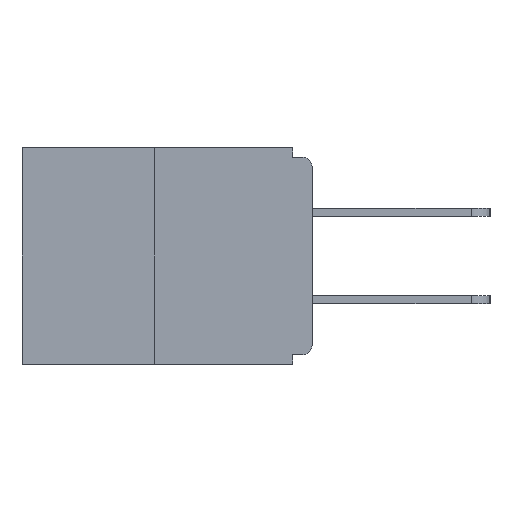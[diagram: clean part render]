
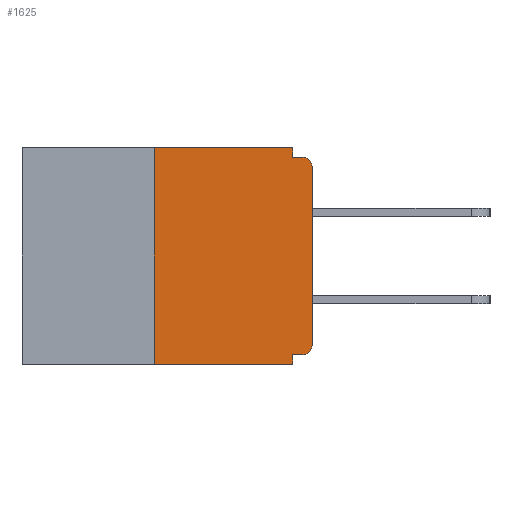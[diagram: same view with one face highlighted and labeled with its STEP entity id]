
A CAD part, left-side view. The second image highlights one B-rep face of the part: STEP entity #1625.
In plain terms, the highlighted planar face has unit normal (-1, 0, 0).
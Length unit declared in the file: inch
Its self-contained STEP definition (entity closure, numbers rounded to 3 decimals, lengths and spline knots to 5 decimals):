
#5 = AXIS2_PLACEMENT_3D ( 'NONE', #1478, #8790, #7945 ) ;
#164 = VECTOR ( 'NONE', #8709, 39.37008 ) ;
#297 = LINE ( 'NONE', #11560, #9770 ) ;
#330 = CARTESIAN_POINT ( 'NONE',  ( 0., 0.25, -0.343 ) ) ;
#506 = VECTOR ( 'NONE', #2333, 39.37008 ) ;
#747 = VERTEX_POINT ( 'NONE', #11713 ) ;
#1061 = CARTESIAN_POINT ( 'NONE',  ( 0., 0.031, 0. ) ) ;
#1192 = CARTESIAN_POINT ( 'NONE',  ( 0., 0.015, -0.313 ) ) ;
#1351 = DIRECTION ( 'NONE',  ( 0., 0., 1. ) ) ;
#1478 = CARTESIAN_POINT ( 'NONE',  ( 0., 0.46, 0. ) ) ;
#1625 = ADVANCED_FACE ( 'NONE', ( #10551 ), #2191, .F. ) ;
#1635 = EDGE_CURVE ( 'NONE', #10508, #9556, #4396, .T. ) ;
#1732 = EDGE_CURVE ( 'NONE', #10364, #5796, #297, .T. ) ;
#1770 = EDGE_CURVE ( 'NONE', #5796, #747, #4181, .T. ) ;
#2173 = CARTESIAN_POINT ( 'NONE',  ( 0., 0., -0.328 ) ) ;
#2191 = PLANE ( 'NONE',  #5 ) ;
#2203 = DIRECTION ( 'NONE',  ( -1., 0., 0. ) ) ;
#2333 = DIRECTION ( 'NONE',  ( 0., -1., 0. ) ) ;
#2385 = CIRCLE ( 'NONE', #3737, 0.015 ) ;
#2574 = LINE ( 'NONE', #2173, #9597 ) ;
#2577 = CARTESIAN_POINT ( 'NONE',  ( 0., 0., -0.015 ) ) ;
#2754 = VECTOR ( 'NONE', #9348, 39.37008 ) ;
#3323 = VERTEX_POINT ( 'NONE', #9105 ) ;
#3351 = EDGE_CURVE ( 'NONE', #7795, #10508, #2574, .T. ) ;
#3388 = CARTESIAN_POINT ( 'NONE',  ( 0., 0.46, -0.343 ) ) ;
#3415 = CARTESIAN_POINT ( 'NONE',  ( 0., 0.031, -0.343 ) ) ;
#3664 = ORIENTED_EDGE ( 'NONE', *, *, #5483, .T. ) ;
#3737 = AXIS2_PLACEMENT_3D ( 'NONE', #10527, #2203, #10576 ) ;
#3806 = VECTOR ( 'NONE', #10780, 39.37008 ) ;
#3870 = EDGE_CURVE ( 'NONE', #7795, #3323, #8283, .T. ) ;
#4018 = VECTOR ( 'NONE', #10853, 39.37008 ) ;
#4101 = CARTESIAN_POINT ( 'NONE',  ( 0., 0.031, -0.343 ) ) ;
#4181 = LINE ( 'NONE', #2577, #4018 ) ;
#4396 = LINE ( 'NONE', #4101, #164 ) ;
#4628 = ORIENTED_EDGE ( 'NONE', *, *, #3870, .T. ) ;
#4729 = DIRECTION ( 'NONE',  ( 0., 0., -1. ) ) ;
#5066 = CARTESIAN_POINT ( 'NONE',  ( 0., 0.25, 0. ) ) ;
#5091 = CARTESIAN_POINT ( 'NONE',  ( 0., 0.46, 0. ) ) ;
#5300 = EDGE_LOOP ( 'NONE', ( #7437, #8618, #5725, #10339, #7276, #4628, #11857, #3664, #6921, #9392 ) ) ;
#5483 = EDGE_CURVE ( 'NONE', #10702, #747, #2385, .T. ) ;
#5725 = ORIENTED_EDGE ( 'NONE', *, *, #8957, .T. ) ;
#5796 = VERTEX_POINT ( 'NONE', #8775 ) ;
#6315 = LINE ( 'NONE', #7747, #6838 ) ;
#6353 = EDGE_CURVE ( 'NONE', #9298, #10775, #6315, .T. ) ;
#6661 = CARTESIAN_POINT ( 'NONE',  ( 0., 0., -0.03 ) ) ;
#6838 = VECTOR ( 'NONE', #1351, 39.37008 ) ;
#6921 = ORIENTED_EDGE ( 'NONE', *, *, #1770, .F. ) ;
#7130 = CARTESIAN_POINT ( 'NONE',  ( 0., 0.015, -0.328 ) ) ;
#7276 = ORIENTED_EDGE ( 'NONE', *, *, #3351, .F. ) ;
#7437 = ORIENTED_EDGE ( 'NONE', *, *, #7565, .F. ) ;
#7491 = CARTESIAN_POINT ( 'NONE',  ( 0., 0., 0. ) ) ;
#7565 = EDGE_CURVE ( 'NONE', #10775, #10364, #10701, .T. ) ;
#7747 = CARTESIAN_POINT ( 'NONE',  ( 0., 0.25, 0. ) ) ;
#7795 = VERTEX_POINT ( 'NONE', #7130 ) ;
#7806 = CARTESIAN_POINT ( 'NONE',  ( 0., 0.031, -0.328 ) ) ;
#7823 = LINE ( 'NONE', #3388, #3806 ) ;
#7945 = DIRECTION ( 'NONE',  ( 0., 0., -1. ) ) ;
#8283 = CIRCLE ( 'NONE', #8385, 0.015 ) ;
#8354 = DIRECTION ( 'NONE',  ( -1., 0., 0. ) ) ;
#8385 = AXIS2_PLACEMENT_3D ( 'NONE', #1192, #8354, #4729 ) ;
#8599 = DIRECTION ( 'NONE',  ( 0., 1., 0. ) ) ;
#8618 = ORIENTED_EDGE ( 'NONE', *, *, #6353, .F. ) ;
#8709 = DIRECTION ( 'NONE',  ( 0., 0., -1. ) ) ;
#8775 = CARTESIAN_POINT ( 'NONE',  ( 0., 0.031, -0.015 ) ) ;
#8790 = DIRECTION ( 'NONE',  ( 1., 0., 0. ) ) ;
#8957 = EDGE_CURVE ( 'NONE', #9298, #9556, #7823, .T. ) ;
#9105 = CARTESIAN_POINT ( 'NONE',  ( 0., 0., -0.313 ) ) ;
#9298 = VERTEX_POINT ( 'NONE', #330 ) ;
#9348 = DIRECTION ( 'NONE',  ( 0., 0., 1. ) ) ;
#9392 = ORIENTED_EDGE ( 'NONE', *, *, #1732, .F. ) ;
#9556 = VERTEX_POINT ( 'NONE', #3415 ) ;
#9597 = VECTOR ( 'NONE', #8599, 39.37008 ) ;
#9770 = VECTOR ( 'NONE', #11606, 39.37008 ) ;
#10339 = ORIENTED_EDGE ( 'NONE', *, *, #1635, .F. ) ;
#10364 = VERTEX_POINT ( 'NONE', #1061 ) ;
#10508 = VERTEX_POINT ( 'NONE', #7806 ) ;
#10527 = CARTESIAN_POINT ( 'NONE',  ( 0., 0.015, -0.03 ) ) ;
#10551 = FACE_OUTER_BOUND ( 'NONE', #5300, .T. ) ;
#10576 = DIRECTION ( 'NONE',  ( 0., 0., -1. ) ) ;
#10663 = EDGE_CURVE ( 'NONE', #3323, #10702, #11649, .T. ) ;
#10701 = LINE ( 'NONE', #5091, #506 ) ;
#10702 = VERTEX_POINT ( 'NONE', #6661 ) ;
#10775 = VERTEX_POINT ( 'NONE', #5066 ) ;
#10780 = DIRECTION ( 'NONE',  ( 0., -1., 0. ) ) ;
#10853 = DIRECTION ( 'NONE',  ( 0., -1., 0. ) ) ;
#11560 = CARTESIAN_POINT ( 'NONE',  ( 0., 0.031, 0. ) ) ;
#11606 = DIRECTION ( 'NONE',  ( 0., 0., -1. ) ) ;
#11649 = LINE ( 'NONE', #7491, #2754 ) ;
#11713 = CARTESIAN_POINT ( 'NONE',  ( 0., 0.015, -0.015 ) ) ;
#11857 = ORIENTED_EDGE ( 'NONE', *, *, #10663, .T. ) ;
